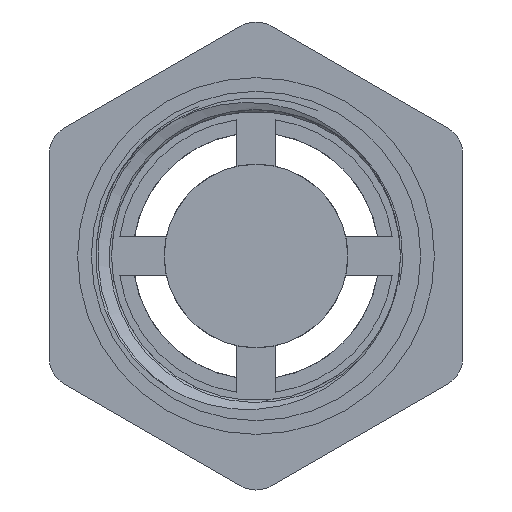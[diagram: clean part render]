
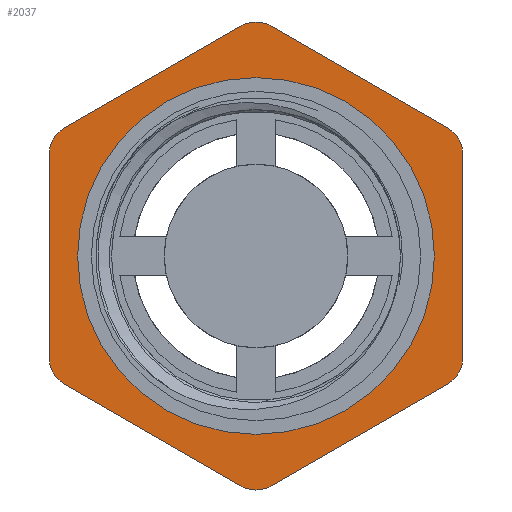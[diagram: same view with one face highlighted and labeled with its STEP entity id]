
A CAD part, front view. The second image highlights one B-rep face of the part: STEP entity #2037.
In plain terms, the highlighted planar face has unit normal (0, -1, 0).
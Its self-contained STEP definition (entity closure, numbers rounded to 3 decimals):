
#35=FACE_BOUND('',#272,.T.);
#66=PLANE('',#2251);
#162=FACE_OUTER_BOUND('',#271,.T.);
#271=EDGE_LOOP('',(#1682,#1683,#1684,#1685,#1686,#1687,#1688,#1689,#1690,
#1691,#1692,#1693));
#272=EDGE_LOOP('',(#1694));
#368=CIRCLE('',#2218,2.);
#376=CIRCLE('',#2231,2.);
#377=CIRCLE('',#2233,2.);
#378=CIRCLE('',#2236,2.);
#379=CIRCLE('',#2238,2.);
#380=CIRCLE('',#2241,2.);
#383=CIRCLE('',#2248,11.672);
#533=LINE('',#3862,#665);
#595=LINE('',#4231,#727);
#596=LINE('',#4233,#728);
#599=LINE('',#4248,#731);
#600=LINE('',#4249,#732);
#601=LINE('',#4250,#733);
#665=VECTOR('',#2455,10.);
#727=VECTOR('',#2715,10.);
#728=VECTOR('',#2718,10.);
#731=VECTOR('',#2737,10.);
#732=VECTOR('',#2738,10.);
#733=VECTOR('',#2739,10.);
#862=VERTEX_POINT('',#3859);
#863=VERTEX_POINT('',#3861);
#921=VERTEX_POINT('',#4181);
#925=VERTEX_POINT('',#4199);
#926=VERTEX_POINT('',#4200);
#927=VERTEX_POINT('',#4205);
#928=VERTEX_POINT('',#4206);
#929=VERTEX_POINT('',#4213);
#930=VERTEX_POINT('',#4214);
#931=VERTEX_POINT('',#4219);
#932=VERTEX_POINT('',#4220);
#933=VERTEX_POINT('',#4227);
#936=VERTEX_POINT('',#4241);
#1095=EDGE_CURVE('',#863,#862,#533,.T.);
#1196=EDGE_CURVE('',#863,#921,#368,.T.);
#1205=EDGE_CURVE('',#925,#926,#376,.T.);
#1208=EDGE_CURVE('',#927,#928,#377,.T.);
#1212=EDGE_CURVE('',#929,#930,#378,.T.);
#1215=EDGE_CURVE('',#931,#932,#379,.T.);
#1219=EDGE_CURVE('',#933,#862,#380,.T.);
#1221=EDGE_CURVE('',#925,#930,#595,.T.);
#1222=EDGE_CURVE('',#929,#921,#596,.T.);
#1226=EDGE_CURVE('',#936,#936,#383,.T.);
#1229=EDGE_CURVE('',#933,#932,#599,.T.);
#1230=EDGE_CURVE('',#931,#928,#600,.T.);
#1231=EDGE_CURVE('',#927,#926,#601,.T.);
#1682=ORIENTED_EDGE('',*,*,#1205,.F.);
#1683=ORIENTED_EDGE('',*,*,#1221,.T.);
#1684=ORIENTED_EDGE('',*,*,#1212,.F.);
#1685=ORIENTED_EDGE('',*,*,#1222,.T.);
#1686=ORIENTED_EDGE('',*,*,#1196,.F.);
#1687=ORIENTED_EDGE('',*,*,#1095,.T.);
#1688=ORIENTED_EDGE('',*,*,#1219,.F.);
#1689=ORIENTED_EDGE('',*,*,#1229,.T.);
#1690=ORIENTED_EDGE('',*,*,#1215,.F.);
#1691=ORIENTED_EDGE('',*,*,#1230,.T.);
#1692=ORIENTED_EDGE('',*,*,#1208,.F.);
#1693=ORIENTED_EDGE('',*,*,#1231,.T.);
#1694=ORIENTED_EDGE('',*,*,#1226,.T.);
#2037=ADVANCED_FACE('',(#162,#35),#66,.T.);
#2218=AXIS2_PLACEMENT_3D('',#4182,#2653,#2654);
#2231=AXIS2_PLACEMENT_3D('',#4201,#2680,#2681);
#2233=AXIS2_PLACEMENT_3D('',#4207,#2686,#2687);
#2236=AXIS2_PLACEMENT_3D('',#4215,#2695,#2696);
#2238=AXIS2_PLACEMENT_3D('',#4221,#2701,#2702);
#2241=AXIS2_PLACEMENT_3D('',#4228,#2710,#2711);
#2248=AXIS2_PLACEMENT_3D('',#4242,#2728,#2729);
#2251=AXIS2_PLACEMENT_3D('',#4247,#2735,#2736);
#2455=DIRECTION('',(0.,0.,1.));
#2653=DIRECTION('center_axis',(0.,1.,0.));
#2654=DIRECTION('ref_axis',(0.866,0.,-0.5));
#2680=DIRECTION('center_axis',(0.,1.,0.));
#2681=DIRECTION('ref_axis',(-0.866,0.,-0.5));
#2686=DIRECTION('center_axis',(0.,1.,0.));
#2687=DIRECTION('ref_axis',(-0.866,0.,0.5));
#2695=DIRECTION('center_axis',(0.,1.,0.));
#2696=DIRECTION('ref_axis',(0.,0.,-1.));
#2701=DIRECTION('center_axis',(0.,1.,0.));
#2702=DIRECTION('ref_axis',(0.,0.,1.));
#2710=DIRECTION('center_axis',(0.,1.,0.));
#2711=DIRECTION('ref_axis',(0.866,0.,0.5));
#2715=DIRECTION('',(0.866,0.,-0.5));
#2718=DIRECTION('',(0.866,0.,0.5));
#2728=DIRECTION('center_axis',(0.,1.,0.));
#2729=DIRECTION('ref_axis',(-1.,0.,0.));
#2735=DIRECTION('center_axis',(0.,-1.,0.));
#2736=DIRECTION('ref_axis',(0.,0.,-1.));
#2737=DIRECTION('',(-0.866,0.,0.5));
#2738=DIRECTION('',(-0.866,0.,-0.5));
#2739=DIRECTION('',(0.,0.,-1.));
#3859=CARTESIAN_POINT('',(13.524,-25.4,6.653));
#3861=CARTESIAN_POINT('',(13.524,-25.4,-6.653));
#3862=CARTESIAN_POINT('',(13.524,-25.4,-7.808));
#4181=CARTESIAN_POINT('',(12.524,-25.4,-8.385));
#4182=CARTESIAN_POINT('Origin',(11.524,-25.4,-6.653));
#4199=CARTESIAN_POINT('',(-12.524,-25.4,-8.385));
#4200=CARTESIAN_POINT('',(-13.524,-25.4,-6.653));
#4201=CARTESIAN_POINT('Origin',(-11.524,-25.4,-6.653));
#4205=CARTESIAN_POINT('',(-13.524,-25.4,6.653));
#4206=CARTESIAN_POINT('',(-12.524,-25.4,8.385));
#4207=CARTESIAN_POINT('Origin',(-11.524,-25.4,6.653));
#4213=CARTESIAN_POINT('',(1.,-25.4,-15.038));
#4214=CARTESIAN_POINT('',(-1.,-25.4,-15.038));
#4215=CARTESIAN_POINT('Origin',(0.,-25.4,-13.306));
#4219=CARTESIAN_POINT('',(-1.,-25.4,15.038));
#4220=CARTESIAN_POINT('',(1.,-25.4,15.038));
#4221=CARTESIAN_POINT('Origin',(0.,-25.4,13.306));
#4227=CARTESIAN_POINT('',(12.524,-25.4,8.385));
#4228=CARTESIAN_POINT('Origin',(11.524,-25.4,6.653));
#4231=CARTESIAN_POINT('',(-13.524,-25.4,-7.808));
#4233=CARTESIAN_POINT('',(0.,-25.4,-15.616));
#4241=CARTESIAN_POINT('',(11.672,-25.4,0.));
#4242=CARTESIAN_POINT('Origin',(0.,-25.4,0.));
#4247=CARTESIAN_POINT('Origin',(0.,-25.4,0.));
#4248=CARTESIAN_POINT('',(13.524,-25.4,7.808));
#4249=CARTESIAN_POINT('',(0.,-25.4,15.616));
#4250=CARTESIAN_POINT('',(-13.524,-25.4,7.808));
